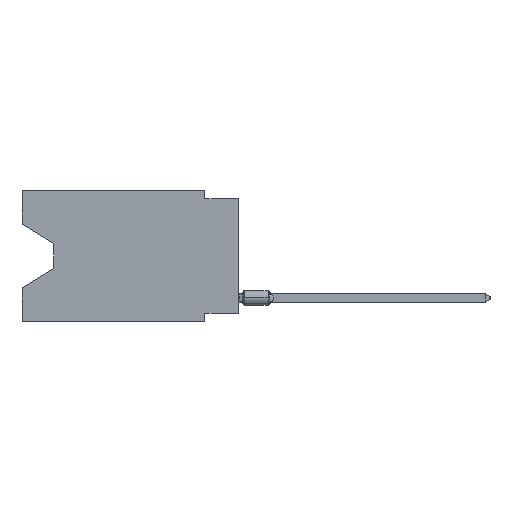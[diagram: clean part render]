
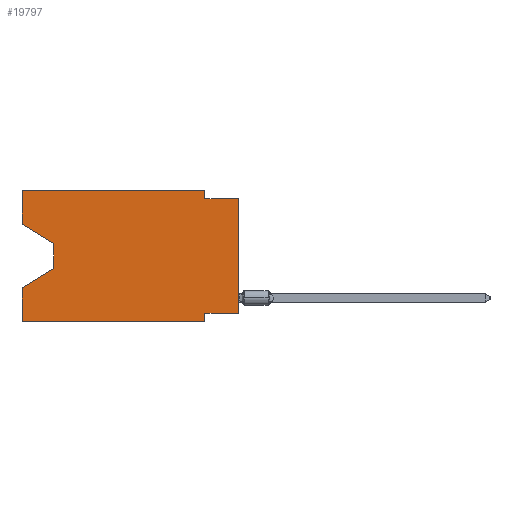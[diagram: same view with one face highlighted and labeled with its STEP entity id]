
A CAD part, left-side view. The second image highlights one B-rep face of the part: STEP entity #19797.
In plain terms, the highlighted planar face has unit normal (-1, 0, 0).
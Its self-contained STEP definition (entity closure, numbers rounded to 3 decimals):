
#823 = VECTOR ( 'NONE', #16232, 1000. ) ;
#844 = CARTESIAN_POINT ( 'NONE',  ( 0., 2.54, -9.906 ) ) ;
#999 = LINE ( 'NONE', #4050, #823 ) ;
#1323 = LINE ( 'NONE', #20438, #11444 ) ;
#1384 = LINE ( 'NONE', #31890, #30552 ) ;
#1803 = DIRECTION ( 'NONE',  ( 0., -1., 0. ) ) ;
#1922 = ORIENTED_EDGE ( 'NONE', *, *, #7611, .F. ) ;
#2206 = FACE_OUTER_BOUND ( 'NONE', #25363, .T. ) ;
#2507 = VECTOR ( 'NONE', #33747, 1000. ) ;
#3207 = EDGE_CURVE ( 'NONE', #15629, #8756, #21614, .T. ) ;
#3327 = ORIENTED_EDGE ( 'NONE', *, *, #11013, .F. ) ;
#3694 = DIRECTION ( 'NONE',  ( 0., 0., -1. ) ) ;
#3768 = VECTOR ( 'NONE', #3694, 1000. ) ;
#4040 = DIRECTION ( 'NONE',  ( 0., 0., 1. ) ) ;
#4050 = CARTESIAN_POINT ( 'NONE',  ( 0., 13.97, -5.893 ) ) ;
#4843 = DIRECTION ( 'NONE',  ( 1., 0., 0. ) ) ;
#5330 = VERTEX_POINT ( 'NONE', #34629 ) ;
#5759 = VECTOR ( 'NONE', #28821, 1000. ) ;
#5869 = VERTEX_POINT ( 'NONE', #9574 ) ;
#6757 = LINE ( 'NONE', #844, #3768 ) ;
#7412 = VERTEX_POINT ( 'NONE', #11958 ) ;
#7611 = EDGE_CURVE ( 'NONE', #34382, #5330, #1323, .T. ) ;
#8679 = EDGE_CURVE ( 'NONE', #33516, #27585, #21147, .T. ) ;
#8756 = VERTEX_POINT ( 'NONE', #15835 ) ;
#9527 = EDGE_CURVE ( 'NONE', #8756, #39116, #6757, .T. ) ;
#9538 = LINE ( 'NONE', #15843, #34045 ) ;
#9574 = CARTESIAN_POINT ( 'NONE',  ( 0., 16.383, -7.36 ) ) ;
#9800 = CARTESIAN_POINT ( 'NONE',  ( 0., 2.54, -9.906 ) ) ;
#9862 = EDGE_CURVE ( 'NONE', #18118, #34382, #36810, .T. ) ;
#10580 = VERTEX_POINT ( 'NONE', #18923 ) ;
#11013 = EDGE_CURVE ( 'NONE', #10580, #24018, #16421, .T. ) ;
#11444 = VECTOR ( 'NONE', #17382, 1000. ) ;
#11958 = CARTESIAN_POINT ( 'NONE',  ( 0., 16.383, -9.906 ) ) ;
#14599 = CARTESIAN_POINT ( 'NONE',  ( 0., 16.383, 0. ) ) ;
#14840 = DIRECTION ( 'NONE',  ( 0., 0., -1. ) ) ;
#15041 = CARTESIAN_POINT ( 'NONE',  ( 0., 13.97, -4.013 ) ) ;
#15629 = VERTEX_POINT ( 'NONE', #33772 ) ;
#15769 = ORIENTED_EDGE ( 'NONE', *, *, #26370, .F. ) ;
#15835 = CARTESIAN_POINT ( 'NONE',  ( 0., 2.54, -9.271 ) ) ;
#15843 = CARTESIAN_POINT ( 'NONE',  ( 0., 0., 0. ) ) ;
#15879 = ORIENTED_EDGE ( 'NONE', *, *, #21838, .T. ) ;
#16232 = DIRECTION ( 'NONE',  ( 0., 0.855, -0.519 ) ) ;
#16421 = LINE ( 'NONE', #17009, #5759 ) ;
#16864 = DIRECTION ( 'NONE',  ( 0., -1., 0. ) ) ;
#17009 = CARTESIAN_POINT ( 'NONE',  ( 0., 16.383, 0. ) ) ;
#17022 = DIRECTION ( 'NONE',  ( 0., 0., -1. ) ) ;
#17382 = DIRECTION ( 'NONE',  ( 0., -1., 0. ) ) ;
#17479 = CARTESIAN_POINT ( 'NONE',  ( 0., 16.383, 0. ) ) ;
#17675 = ORIENTED_EDGE ( 'NONE', *, *, #24673, .T. ) ;
#18020 = VECTOR ( 'NONE', #14840, 1000. ) ;
#18118 = VERTEX_POINT ( 'NONE', #39266 ) ;
#18564 = CARTESIAN_POINT ( 'NONE',  ( 0., 0., -9.271 ) ) ;
#18923 = CARTESIAN_POINT ( 'NONE',  ( 0., 16.383, -2.546 ) ) ;
#19797 = ADVANCED_FACE ( 'NONE', ( #2206 ), #33302, .F. ) ;
#20438 = CARTESIAN_POINT ( 'NONE',  ( 0., 0., -0.635 ) ) ;
#20824 = EDGE_CURVE ( 'NONE', #27585, #5869, #999, .T. ) ;
#21147 = LINE ( 'NONE', #15041, #18020 ) ;
#21267 = DIRECTION ( 'NONE',  ( 0., -0.855, -0.519 ) ) ;
#21345 = CARTESIAN_POINT ( 'NONE',  ( 0., 2.54, 0. ) ) ;
#21397 = ORIENTED_EDGE ( 'NONE', *, *, #3207, .F. ) ;
#21614 = LINE ( 'NONE', #18564, #29370 ) ;
#21838 = EDGE_CURVE ( 'NONE', #15629, #5330, #9538, .T. ) ;
#22556 = ORIENTED_EDGE ( 'NONE', *, *, #9527, .F. ) ;
#22833 = CARTESIAN_POINT ( 'NONE',  ( 0., 13.97, -4.013 ) ) ;
#23144 = EDGE_CURVE ( 'NONE', #7412, #5869, #28091, .T. ) ;
#23270 = CARTESIAN_POINT ( 'NONE',  ( 0., 16.383, 0. ) ) ;
#24018 = VERTEX_POINT ( 'NONE', #23270 ) ;
#24510 = ORIENTED_EDGE ( 'NONE', *, *, #23144, .F. ) ;
#24673 = EDGE_CURVE ( 'NONE', #7412, #39116, #1384, .T. ) ;
#25363 = EDGE_LOOP ( 'NONE', ( #26103, #37018, #37633, #24510, #17675, #22556, #21397, #15879, #1922, #33047, #15769, #3327 ) ) ;
#26103 = ORIENTED_EDGE ( 'NONE', *, *, #32449, .T. ) ;
#26370 = EDGE_CURVE ( 'NONE', #24018, #18118, #32314, .T. ) ;
#26954 = CARTESIAN_POINT ( 'NONE',  ( 0., 2.54, -0.635 ) ) ;
#27585 = VERTEX_POINT ( 'NONE', #32125 ) ;
#28091 = LINE ( 'NONE', #30347, #33188 ) ;
#28821 = DIRECTION ( 'NONE',  ( 0., 0., 1. ) ) ;
#29370 = VECTOR ( 'NONE', #36882, 1000. ) ;
#29516 = VECTOR ( 'NONE', #21267, 1000. ) ;
#30347 = CARTESIAN_POINT ( 'NONE',  ( 0., 16.383, 0. ) ) ;
#30552 = VECTOR ( 'NONE', #1803, 1000. ) ;
#31194 = CARTESIAN_POINT ( 'NONE',  ( 0., 16.383, -2.546 ) ) ;
#31890 = CARTESIAN_POINT ( 'NONE',  ( 0., 16.383, -9.906 ) ) ;
#32125 = CARTESIAN_POINT ( 'NONE',  ( 0., 13.97, -5.893 ) ) ;
#32314 = LINE ( 'NONE', #17479, #39095 ) ;
#32449 = EDGE_CURVE ( 'NONE', #10580, #33516, #34074, .T. ) ;
#32547 = AXIS2_PLACEMENT_3D ( 'NONE', #14599, #4843, #17022 ) ;
#33047 = ORIENTED_EDGE ( 'NONE', *, *, #9862, .F. ) ;
#33188 = VECTOR ( 'NONE', #33416, 1000. ) ;
#33302 = PLANE ( 'NONE',  #32547 ) ;
#33416 = DIRECTION ( 'NONE',  ( 0., 0., 1. ) ) ;
#33516 = VERTEX_POINT ( 'NONE', #22833 ) ;
#33747 = DIRECTION ( 'NONE',  ( 0., 0., -1. ) ) ;
#33772 = CARTESIAN_POINT ( 'NONE',  ( 0., 0., -9.271 ) ) ;
#34045 = VECTOR ( 'NONE', #4040, 1000. ) ;
#34074 = LINE ( 'NONE', #31194, #29516 ) ;
#34382 = VERTEX_POINT ( 'NONE', #26954 ) ;
#34629 = CARTESIAN_POINT ( 'NONE',  ( 0., 0., -0.635 ) ) ;
#36810 = LINE ( 'NONE', #21345, #2507 ) ;
#36882 = DIRECTION ( 'NONE',  ( 0., 1., 0. ) ) ;
#37018 = ORIENTED_EDGE ( 'NONE', *, *, #8679, .T. ) ;
#37633 = ORIENTED_EDGE ( 'NONE', *, *, #20824, .T. ) ;
#39095 = VECTOR ( 'NONE', #16864, 1000. ) ;
#39116 = VERTEX_POINT ( 'NONE', #9800 ) ;
#39266 = CARTESIAN_POINT ( 'NONE',  ( 0., 2.54, 0. ) ) ;
